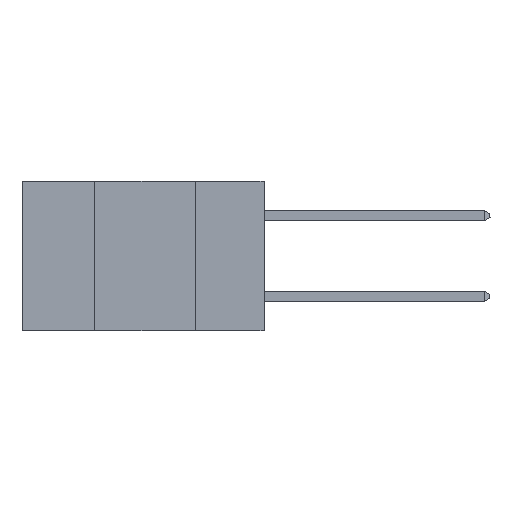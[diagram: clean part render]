
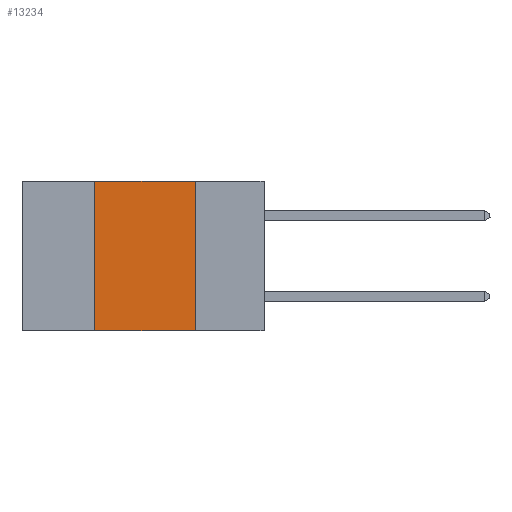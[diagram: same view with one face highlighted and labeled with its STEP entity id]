
A CAD part, left-side view. The second image highlights one B-rep face of the part: STEP entity #13234.
In plain terms, the highlighted planar face has unit normal (-1, 0, 0).
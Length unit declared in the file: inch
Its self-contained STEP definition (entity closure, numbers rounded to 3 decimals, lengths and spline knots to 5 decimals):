
#70 = CARTESIAN_POINT ( 'NONE',  ( 0., 0.6, -0.37 ) ) ;
#679 = LINE ( 'NONE', #11943, #10083 ) ;
#1543 = VECTOR ( 'NONE', #12627, 39.37008 ) ;
#2167 = CARTESIAN_POINT ( 'NONE',  ( 0., 0.17, 0. ) ) ;
#3066 = LINE ( 'NONE', #8698, #1543 ) ;
#3745 = VECTOR ( 'NONE', #8010, 39.37008 ) ;
#3809 = ORIENTED_EDGE ( 'NONE', *, *, #14915, .F. ) ;
#3877 = DIRECTION ( 'NONE',  ( 0., -1., 0. ) ) ;
#5272 = AXIS2_PLACEMENT_3D ( 'NONE', #10242, #12632, #6499 ) ;
#5663 = DIRECTION ( 'NONE',  ( 0., -1., 0. ) ) ;
#6499 = DIRECTION ( 'NONE',  ( 0., 0., -1. ) ) ;
#6546 = CARTESIAN_POINT ( 'NONE',  ( 0., 0.17, -0.37 ) ) ;
#7933 = FACE_OUTER_BOUND ( 'NONE', #12277, .T. ) ;
#8010 = DIRECTION ( 'NONE',  ( 0., 0., -1. ) ) ;
#8281 = VERTEX_POINT ( 'NONE', #2167 ) ;
#8344 = EDGE_CURVE ( 'NONE', #10558, #13563, #10915, .T. ) ;
#8563 = LINE ( 'NONE', #10597, #3745 ) ;
#8637 = EDGE_CURVE ( 'NONE', #10558, #9360, #3066, .T. ) ;
#8698 = CARTESIAN_POINT ( 'NONE',  ( 0., 0.42, 0. ) ) ;
#9074 = ORIENTED_EDGE ( 'NONE', *, *, #10996, .F. ) ;
#9360 = VERTEX_POINT ( 'NONE', #13934 ) ;
#10083 = VECTOR ( 'NONE', #5663, 39.37008 ) ;
#10242 = CARTESIAN_POINT ( 'NONE',  ( 0., 0.6, 0. ) ) ;
#10553 = ORIENTED_EDGE ( 'NONE', *, *, #8637, .F. ) ;
#10558 = VERTEX_POINT ( 'NONE', #15443 ) ;
#10597 = CARTESIAN_POINT ( 'NONE',  ( 0., 0.17, 0. ) ) ;
#10915 = LINE ( 'NONE', #70, #11896 ) ;
#10996 = EDGE_CURVE ( 'NONE', #9360, #8281, #679, .T. ) ;
#11372 = PLANE ( 'NONE',  #5272 ) ;
#11896 = VECTOR ( 'NONE', #3877, 39.37008 ) ;
#11943 = CARTESIAN_POINT ( 'NONE',  ( 0., 0.6, 0. ) ) ;
#12277 = EDGE_LOOP ( 'NONE', ( #3809, #9074, #10553, #15265 ) ) ;
#12627 = DIRECTION ( 'NONE',  ( 0., 0., 1. ) ) ;
#12632 = DIRECTION ( 'NONE',  ( 1., 0., 0. ) ) ;
#13234 = ADVANCED_FACE ( 'NONE', ( #7933 ), #11372, .F. ) ;
#13563 = VERTEX_POINT ( 'NONE', #6546 ) ;
#13934 = CARTESIAN_POINT ( 'NONE',  ( 0., 0.42, 0. ) ) ;
#14915 = EDGE_CURVE ( 'NONE', #8281, #13563, #8563, .T. ) ;
#15265 = ORIENTED_EDGE ( 'NONE', *, *, #8344, .T. ) ;
#15443 = CARTESIAN_POINT ( 'NONE',  ( 0., 0.42, -0.37 ) ) ;
